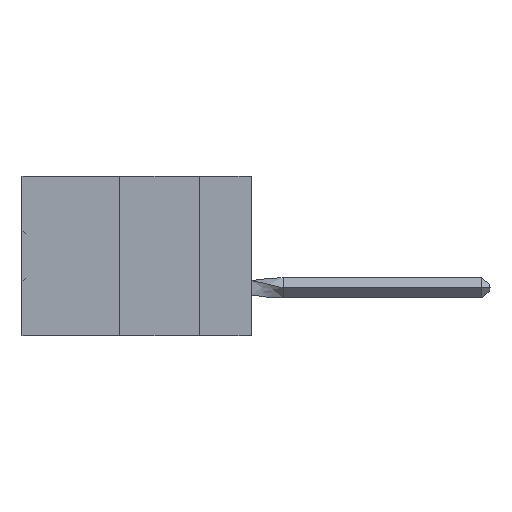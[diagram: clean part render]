
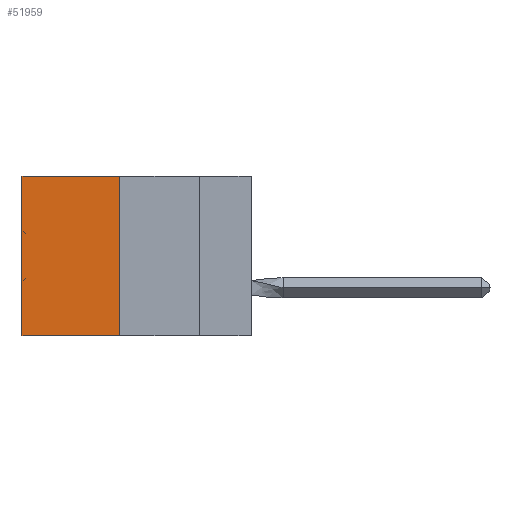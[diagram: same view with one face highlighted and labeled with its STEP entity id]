
A CAD part, left-side view. The second image highlights one B-rep face of the part: STEP entity #51959.
In plain terms, the highlighted planar face has unit normal (-1, 0, 0).
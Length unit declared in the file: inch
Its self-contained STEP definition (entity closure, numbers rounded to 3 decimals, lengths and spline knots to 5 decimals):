
#2792 = CARTESIAN_POINT ( 'NONE',  ( 0.305, 0.72, -0.5 ) ) ;
#2883 = PLANE ( 'NONE',  #3458 ) ;
#3458 = AXIS2_PLACEMENT_3D ( 'NONE', #20727, #33515, #38420 ) ;
#5292 = VECTOR ( 'NONE', #35920, 39.37008 ) ;
#6638 = CARTESIAN_POINT ( 'NONE',  ( 0.305, 0.413, -0.5 ) ) ;
#7688 = VERTEX_POINT ( 'NONE', #24538 ) ;
#8477 = LINE ( 'NONE', #20256, #33933 ) ;
#9963 = VERTEX_POINT ( 'NONE', #6638 ) ;
#11419 = EDGE_CURVE ( 'NONE', #11522, #51516, #50629, .T. ) ;
#11522 = VERTEX_POINT ( 'NONE', #41303 ) ;
#12428 = EDGE_CURVE ( 'NONE', #11522, #9963, #31362, .T. ) ;
#13100 = ORIENTED_EDGE ( 'NONE', *, *, #12428, .F. ) ;
#13617 = CARTESIAN_POINT ( 'NONE',  ( 0.305, 0.413, 0. ) ) ;
#16022 = VECTOR ( 'NONE', #46968, 39.37008 ) ;
#17398 = DIRECTION ( 'NONE',  ( 0., 0., -1. ) ) ;
#20256 = CARTESIAN_POINT ( 'NONE',  ( 0.305, 0.413, -0.5 ) ) ;
#20727 = CARTESIAN_POINT ( 'NONE',  ( 0.305, 0.413, -0.5 ) ) ;
#20977 = EDGE_CURVE ( 'NONE', #9963, #7688, #8477, .T. ) ;
#22260 = EDGE_LOOP ( 'NONE', ( #29850, #27492, #13100, #54339 ) ) ;
#22566 = FACE_OUTER_BOUND ( 'NONE', #22260, .T. ) ;
#24371 = DIRECTION ( 'NONE',  ( 0., 1., 0. ) ) ;
#24538 = CARTESIAN_POINT ( 'NONE',  ( 0.305, 0.72, -0.5 ) ) ;
#26974 = CARTESIAN_POINT ( 'NONE',  ( 0.305, 0.72, 0. ) ) ;
#27492 = ORIENTED_EDGE ( 'NONE', *, *, #20977, .F. ) ;
#29850 = ORIENTED_EDGE ( 'NONE', *, *, #49057, .T. ) ;
#29963 = VECTOR ( 'NONE', #17398, 39.37008 ) ;
#31362 = LINE ( 'NONE', #34545, #29963 ) ;
#33515 = DIRECTION ( 'NONE',  ( 1., 0., 0. ) ) ;
#33933 = VECTOR ( 'NONE', #24371, 39.37008 ) ;
#34545 = CARTESIAN_POINT ( 'NONE',  ( 0.305, 0.413, -0.5 ) ) ;
#35920 = DIRECTION ( 'NONE',  ( 0., 1., 0. ) ) ;
#38420 = DIRECTION ( 'NONE',  ( 0., 0., -1. ) ) ;
#39448 = LINE ( 'NONE', #2792, #16022 ) ;
#41303 = CARTESIAN_POINT ( 'NONE',  ( 0.305, 0.413, 0. ) ) ;
#46968 = DIRECTION ( 'NONE',  ( 0., 0., -1. ) ) ;
#49057 = EDGE_CURVE ( 'NONE', #51516, #7688, #39448, .T. ) ;
#50629 = LINE ( 'NONE', #13617, #5292 ) ;
#51516 = VERTEX_POINT ( 'NONE', #26974 ) ;
#51959 = ADVANCED_FACE ( 'NONE', ( #22566 ), #2883, .F. ) ;
#54339 = ORIENTED_EDGE ( 'NONE', *, *, #11419, .T. ) ;
